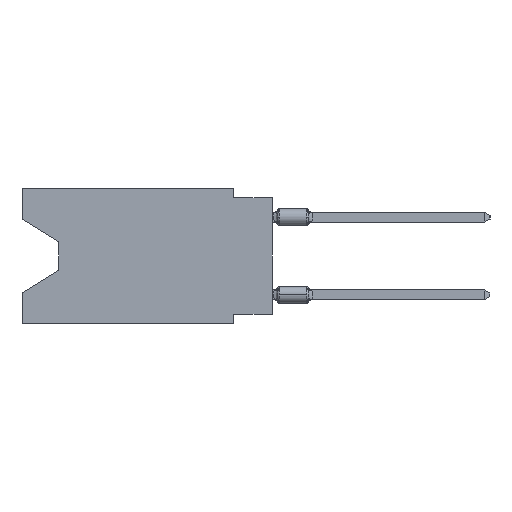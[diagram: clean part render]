
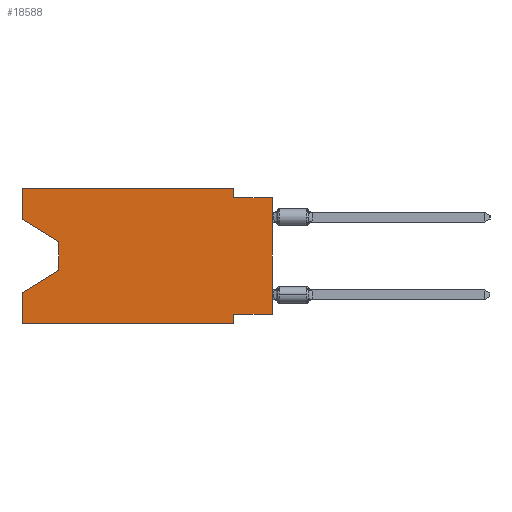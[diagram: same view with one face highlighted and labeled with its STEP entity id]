
A CAD part, left-side view. The second image highlights one B-rep face of the part: STEP entity #18588.
In plain terms, the highlighted planar face has unit normal (-1, 0, 0).
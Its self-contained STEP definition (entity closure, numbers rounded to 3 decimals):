
#89 = CARTESIAN_POINT ( 'NONE',  ( 0., 16.383, 0. ) ) ;
#105 = DIRECTION ( 'NONE',  ( 0., -0.855, -0.519 ) ) ;
#224 = ORIENTED_EDGE ( 'NONE', *, *, #25878, .T. ) ;
#466 = CARTESIAN_POINT ( 'NONE',  ( 0., 16.383, 0. ) ) ;
#991 = DIRECTION ( 'NONE',  ( 0., 0., 1. ) ) ;
#1222 = DIRECTION ( 'NONE',  ( 0., 0., 1. ) ) ;
#1268 = CARTESIAN_POINT ( 'NONE',  ( 0., 13.97, -3.505 ) ) ;
#1414 = CARTESIAN_POINT ( 'NONE',  ( 0., 13.97, -5.385 ) ) ;
#1824 = LINE ( 'NONE', #9956, #15215 ) ;
#2198 = EDGE_LOOP ( 'NONE', ( #12593, #9878, #7739, #25776, #224, #11104, #11633, #25547, #7097, #21422, #22990, #6211 ) ) ;
#2830 = CARTESIAN_POINT ( 'NONE',  ( 0., 0., 0. ) ) ;
#2987 = LINE ( 'NONE', #20953, #6574 ) ;
#3881 = LINE ( 'NONE', #8009, #7827 ) ;
#4151 = EDGE_CURVE ( 'NONE', #19962, #23797, #13640, .T. ) ;
#4735 = VECTOR ( 'NONE', #9414, 1000. ) ;
#4744 = VERTEX_POINT ( 'NONE', #14363 ) ;
#4757 = VECTOR ( 'NONE', #23956, 1000. ) ;
#5334 = VERTEX_POINT ( 'NONE', #16988 ) ;
#5422 = CARTESIAN_POINT ( 'NONE',  ( 0., 0., -8.255 ) ) ;
#5721 = VERTEX_POINT ( 'NONE', #21221 ) ;
#6211 = ORIENTED_EDGE ( 'NONE', *, *, #7111, .F. ) ;
#6488 = LINE ( 'NONE', #14614, #4735 ) ;
#6495 = VERTEX_POINT ( 'NONE', #13140 ) ;
#6574 = VECTOR ( 'NONE', #991, 1000. ) ;
#7037 = CARTESIAN_POINT ( 'NONE',  ( 0., 2.54, 0. ) ) ;
#7097 = ORIENTED_EDGE ( 'NONE', *, *, #22650, .F. ) ;
#7111 = EDGE_CURVE ( 'NONE', #21886, #12036, #3881, .T. ) ;
#7113 = DIRECTION ( 'NONE',  ( 0., -1., 0. ) ) ;
#7539 = DIRECTION ( 'NONE',  ( 0., 0.855, -0.519 ) ) ;
#7678 = VERTEX_POINT ( 'NONE', #9567 ) ;
#7739 = ORIENTED_EDGE ( 'NONE', *, *, #13492, .T. ) ;
#7755 = DIRECTION ( 'NONE',  ( 0., 0., 1. ) ) ;
#7827 = VECTOR ( 'NONE', #7755, 1000. ) ;
#7964 = DIRECTION ( 'NONE',  ( 0., 0., -1. ) ) ;
#8006 = VECTOR ( 'NONE', #7964, 1000. ) ;
#8009 = CARTESIAN_POINT ( 'NONE',  ( 0., 16.383, 0. ) ) ;
#8012 = EDGE_CURVE ( 'NONE', #5721, #7678, #2987, .T. ) ;
#8586 = DIRECTION ( 'NONE',  ( 1., 0., 0. ) ) ;
#9250 = CARTESIAN_POINT ( 'NONE',  ( 0., 16.383, -8.89 ) ) ;
#9414 = DIRECTION ( 'NONE',  ( 0., -1., 0. ) ) ;
#9567 = CARTESIAN_POINT ( 'NONE',  ( 0., 16.383, -6.852 ) ) ;
#9795 = LINE ( 'NONE', #13514, #16879 ) ;
#9869 = AXIS2_PLACEMENT_3D ( 'NONE', #466, #8586, #16566 ) ;
#9878 = ORIENTED_EDGE ( 'NONE', *, *, #23965, .T. ) ;
#9956 = CARTESIAN_POINT ( 'NONE',  ( 0., 13.97, -3.505 ) ) ;
#10472 = VECTOR ( 'NONE', #7539, 1000. ) ;
#10495 = EDGE_CURVE ( 'NONE', #12036, #18371, #6488, .T. ) ;
#11104 = ORIENTED_EDGE ( 'NONE', *, *, #20923, .F. ) ;
#11277 = VECTOR ( 'NONE', #1222, 1000. ) ;
#11633 = ORIENTED_EDGE ( 'NONE', *, *, #4151, .F. ) ;
#12036 = VERTEX_POINT ( 'NONE', #89 ) ;
#12593 = ORIENTED_EDGE ( 'NONE', *, *, #20957, .T. ) ;
#13140 = CARTESIAN_POINT ( 'NONE',  ( 0., 0., -0.635 ) ) ;
#13282 = VECTOR ( 'NONE', #21630, 1000. ) ;
#13336 = LINE ( 'NONE', #2830, #11277 ) ;
#13492 = EDGE_CURVE ( 'NONE', #5334, #7678, #14880, .T. ) ;
#13514 = CARTESIAN_POINT ( 'NONE',  ( 0., 0., -0.635 ) ) ;
#13640 = LINE ( 'NONE', #15909, #13282 ) ;
#13944 = DIRECTION ( 'NONE',  ( 0., 0., -1. ) ) ;
#14116 = CARTESIAN_POINT ( 'NONE',  ( 0., 2.54, 0. ) ) ;
#14358 = EDGE_CURVE ( 'NONE', #19962, #6495, #13336, .T. ) ;
#14363 = CARTESIAN_POINT ( 'NONE',  ( 0., 2.54, -8.89 ) ) ;
#14614 = CARTESIAN_POINT ( 'NONE',  ( 0., 16.383, 0. ) ) ;
#14880 = LINE ( 'NONE', #1414, #10472 ) ;
#15215 = VECTOR ( 'NONE', #13944, 1000. ) ;
#15490 = LINE ( 'NONE', #9250, #15716 ) ;
#15716 = VECTOR ( 'NONE', #7113, 1000. ) ;
#15909 = CARTESIAN_POINT ( 'NONE',  ( 0., 0., -8.255 ) ) ;
#16152 = CARTESIAN_POINT ( 'NONE',  ( 0., 2.54, -0.635 ) ) ;
#16348 = CARTESIAN_POINT ( 'NONE',  ( 0., 16.383, -2.038 ) ) ;
#16431 = EDGE_CURVE ( 'NONE', #18371, #24406, #26197, .T. ) ;
#16441 = FACE_OUTER_BOUND ( 'NONE', #2198, .T. ) ;
#16566 = DIRECTION ( 'NONE',  ( 0., 0., -1. ) ) ;
#16599 = CARTESIAN_POINT ( 'NONE',  ( 0., 2.54, -8.89 ) ) ;
#16879 = VECTOR ( 'NONE', #25465, 1000. ) ;
#16988 = CARTESIAN_POINT ( 'NONE',  ( 0., 13.97, -5.385 ) ) ;
#18325 = LINE ( 'NONE', #16348, #24567 ) ;
#18371 = VERTEX_POINT ( 'NONE', #7037 ) ;
#18588 = ADVANCED_FACE ( 'NONE', ( #16441 ), #24943, .F. ) ;
#19962 = VERTEX_POINT ( 'NONE', #5422 ) ;
#20923 = EDGE_CURVE ( 'NONE', #23797, #4744, #22079, .T. ) ;
#20953 = CARTESIAN_POINT ( 'NONE',  ( 0., 16.383, 0. ) ) ;
#20957 = EDGE_CURVE ( 'NONE', #21886, #21596, #18325, .T. ) ;
#21221 = CARTESIAN_POINT ( 'NONE',  ( 0., 16.383, -8.89 ) ) ;
#21340 = CARTESIAN_POINT ( 'NONE',  ( 0., 16.383, -2.038 ) ) ;
#21422 = ORIENTED_EDGE ( 'NONE', *, *, #16431, .F. ) ;
#21596 = VERTEX_POINT ( 'NONE', #1268 ) ;
#21630 = DIRECTION ( 'NONE',  ( 0., 1., 0. ) ) ;
#21886 = VERTEX_POINT ( 'NONE', #21340 ) ;
#22079 = LINE ( 'NONE', #16599, #8006 ) ;
#22650 = EDGE_CURVE ( 'NONE', #24406, #6495, #9795, .T. ) ;
#22990 = ORIENTED_EDGE ( 'NONE', *, *, #10495, .F. ) ;
#23797 = VERTEX_POINT ( 'NONE', #25490 ) ;
#23956 = DIRECTION ( 'NONE',  ( 0., 0., -1. ) ) ;
#23965 = EDGE_CURVE ( 'NONE', #21596, #5334, #1824, .T. ) ;
#24406 = VERTEX_POINT ( 'NONE', #16152 ) ;
#24567 = VECTOR ( 'NONE', #105, 1000. ) ;
#24943 = PLANE ( 'NONE',  #9869 ) ;
#25465 = DIRECTION ( 'NONE',  ( 0., -1., 0. ) ) ;
#25490 = CARTESIAN_POINT ( 'NONE',  ( 0., 2.54, -8.255 ) ) ;
#25547 = ORIENTED_EDGE ( 'NONE', *, *, #14358, .T. ) ;
#25776 = ORIENTED_EDGE ( 'NONE', *, *, #8012, .F. ) ;
#25878 = EDGE_CURVE ( 'NONE', #5721, #4744, #15490, .T. ) ;
#26197 = LINE ( 'NONE', #14116, #4757 ) ;
